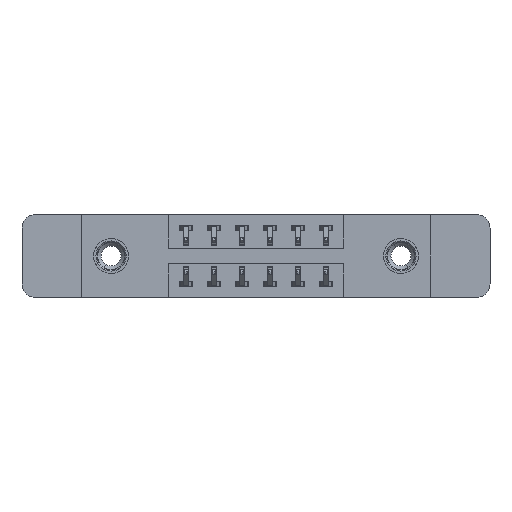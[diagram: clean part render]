
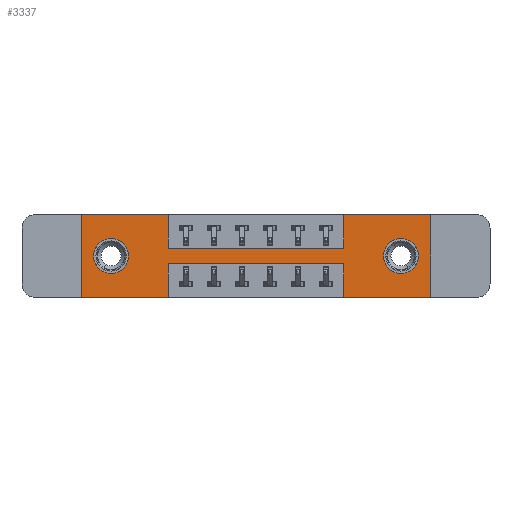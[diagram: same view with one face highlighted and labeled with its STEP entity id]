
A CAD part, front view. The second image highlights one B-rep face of the part: STEP entity #3337.
In plain terms, the highlighted planar face has unit normal (0, -1, 0).
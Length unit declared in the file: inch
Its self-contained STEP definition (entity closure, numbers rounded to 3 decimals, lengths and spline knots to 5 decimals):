
#36 = CARTESIAN_POINT ( 'NONE',  ( 1.1725, 0., -0.22 ) ) ;
#124 = AXIS2_PLACEMENT_3D ( 'NONE', #2717, #1734, #13635 ) ;
#217 = FACE_BOUND ( 'NONE', #1406, .T. ) ;
#240 = AXIS2_PLACEMENT_3D ( 'NONE', #813, #13958, #3029 ) ;
#244 = LINE ( 'NONE', #4098, #6102 ) ;
#320 = CARTESIAN_POINT ( 'NONE',  ( 1.1725, 0., -0.37 ) ) ;
#406 = LINE ( 'NONE', #913, #5225 ) ;
#577 = ORIENTED_EDGE ( 'NONE', *, *, #9553, .F. ) ;
#578 = CARTESIAN_POINT ( 'NONE',  ( 0., 0., -0.37 ) ) ;
#588 = LINE ( 'NONE', #1889, #13231 ) ;
#661 = LINE ( 'NONE', #10753, #5142 ) ;
#663 = ORIENTED_EDGE ( 'NONE', *, *, #7709, .F. ) ;
#774 = DIRECTION ( 'NONE',  ( 1., 0., 0. ) ) ;
#813 = CARTESIAN_POINT ( 'NONE',  ( 1.4275, 0., -0.185 ) ) ;
#877 = DIRECTION ( 'NONE',  ( 0., 0., 1. ) ) ;
#913 = CARTESIAN_POINT ( 'NONE',  ( 1.1725, 0., -0.37 ) ) ;
#930 = VECTOR ( 'NONE', #5246, 39.37008 ) ;
#980 = LINE ( 'NONE', #2436, #3235 ) ;
#1031 = DIRECTION ( 'NONE',  ( -1., 0., 0. ) ) ;
#1097 = LINE ( 'NONE', #12730, #930 ) ;
#1406 = EDGE_LOOP ( 'NONE', ( #3164, #3197 ) ) ;
#1559 = LINE ( 'NONE', #4220, #3796 ) ;
#1603 = PLANE ( 'NONE',  #124 ) ;
#1734 = DIRECTION ( 'NONE',  ( 0., -1., 0. ) ) ;
#1872 = EDGE_CURVE ( 'NONE', #7297, #12879, #4726, .T. ) ;
#1889 = CARTESIAN_POINT ( 'NONE',  ( 1.1725, 0., 0. ) ) ;
#2072 = VERTEX_POINT ( 'NONE', #320 ) ;
#2246 = VECTOR ( 'NONE', #11998, 39.37008 ) ;
#2436 = CARTESIAN_POINT ( 'NONE',  ( 0., 0., -0.37 ) ) ;
#2717 = CARTESIAN_POINT ( 'NONE',  ( 0., 0., -0.37 ) ) ;
#2757 = LINE ( 'NONE', #8033, #12459 ) ;
#2758 = CIRCLE ( 'NONE', #240, 0.078 ) ;
#2958 = VERTEX_POINT ( 'NONE', #13514 ) ;
#3029 = DIRECTION ( 'NONE',  ( 0., 0., -1. ) ) ;
#3122 = ORIENTED_EDGE ( 'NONE', *, *, #12775, .T. ) ;
#3164 = ORIENTED_EDGE ( 'NONE', *, *, #4506, .T. ) ;
#3196 = CARTESIAN_POINT ( 'NONE',  ( 0., 0., 0. ) ) ;
#3197 = ORIENTED_EDGE ( 'NONE', *, *, #11159, .T. ) ;
#3235 = VECTOR ( 'NONE', #7865, 39.37008 ) ;
#3301 = FACE_OUTER_BOUND ( 'NONE', #11328, .T. ) ;
#3337 = ADVANCED_FACE ( 'NONE', ( #217, #10773, #3301 ), #1603, .T. ) ;
#3426 = ORIENTED_EDGE ( 'NONE', *, *, #11419, .F. ) ;
#3471 = DIRECTION ( 'NONE',  ( 0., 1., 0. ) ) ;
#3548 = AXIS2_PLACEMENT_3D ( 'NONE', #3570, #13482, #5794 ) ;
#3570 = CARTESIAN_POINT ( 'NONE',  ( 1.4275, 0., -0.185 ) ) ;
#3595 = CARTESIAN_POINT ( 'NONE',  ( 1.1725, 0., -0.15 ) ) ;
#3692 = VECTOR ( 'NONE', #6111, 39.37008 ) ;
#3796 = VECTOR ( 'NONE', #12183, 39.37008 ) ;
#3921 = EDGE_CURVE ( 'NONE', #5388, #12815, #11264, .T. ) ;
#3966 = DIRECTION ( 'NONE',  ( 1., 0., 0. ) ) ;
#4052 = EDGE_CURVE ( 'NONE', #13413, #6311, #1559, .T. ) ;
#4098 = CARTESIAN_POINT ( 'NONE',  ( 0., 0., 0. ) ) ;
#4147 = CARTESIAN_POINT ( 'NONE',  ( 0.3875, 0., -0.37 ) ) ;
#4220 = CARTESIAN_POINT ( 'NONE',  ( 1.56, 0., 0. ) ) ;
#4366 = VERTEX_POINT ( 'NONE', #7771 ) ;
#4392 = CIRCLE ( 'NONE', #3548, 0.078 ) ;
#4485 = EDGE_CURVE ( 'NONE', #5446, #2958, #8741, .T. ) ;
#4506 = EDGE_CURVE ( 'NONE', #12605, #4366, #2758, .T. ) ;
#4726 = CIRCLE ( 'NONE', #9571, 0.078 ) ;
#4784 = CARTESIAN_POINT ( 'NONE',  ( 1.56, 0., -0.37 ) ) ;
#5142 = VECTOR ( 'NONE', #1031, 39.37008 ) ;
#5225 = VECTOR ( 'NONE', #10772, 39.37008 ) ;
#5246 = DIRECTION ( 'NONE',  ( 0., 0., -1. ) ) ;
#5388 = VERTEX_POINT ( 'NONE', #36 ) ;
#5446 = VERTEX_POINT ( 'NONE', #13851 ) ;
#5616 = VERTEX_POINT ( 'NONE', #3595 ) ;
#5794 = DIRECTION ( 'NONE',  ( 0., 0., -1. ) ) ;
#5885 = ORIENTED_EDGE ( 'NONE', *, *, #8871, .F. ) ;
#5951 = CARTESIAN_POINT ( 'NONE',  ( 0.3875, 0., 0. ) ) ;
#6102 = VECTOR ( 'NONE', #774, 39.37008 ) ;
#6111 = DIRECTION ( 'NONE',  ( 1., 0., 0. ) ) ;
#6289 = CARTESIAN_POINT ( 'NONE',  ( 0., 0., 0. ) ) ;
#6311 = VERTEX_POINT ( 'NONE', #4784 ) ;
#6320 = LINE ( 'NONE', #6289, #11874 ) ;
#6449 = CARTESIAN_POINT ( 'NONE',  ( 0.3875, 0., -0.22 ) ) ;
#6675 = ORIENTED_EDGE ( 'NONE', *, *, #4485, .F. ) ;
#6899 = ORIENTED_EDGE ( 'NONE', *, *, #8560, .F. ) ;
#7297 = VERTEX_POINT ( 'NONE', #13459 ) ;
#7414 = DIRECTION ( 'NONE',  ( 0., 0., -1. ) ) ;
#7482 = CARTESIAN_POINT ( 'NONE',  ( 0.1325, 0., -0.185 ) ) ;
#7622 = DIRECTION ( 'NONE',  ( 0., 0., 1. ) ) ;
#7688 = ORIENTED_EDGE ( 'NONE', *, *, #3921, .F. ) ;
#7709 = EDGE_CURVE ( 'NONE', #13594, #8801, #2757, .T. ) ;
#7771 = CARTESIAN_POINT ( 'NONE',  ( 1.4275, 0., -0.263 ) ) ;
#7865 = DIRECTION ( 'NONE',  ( -1., 0., 0. ) ) ;
#7995 = ORIENTED_EDGE ( 'NONE', *, *, #11277, .F. ) ;
#8033 = CARTESIAN_POINT ( 'NONE',  ( 0., 0., 0. ) ) ;
#8186 = CARTESIAN_POINT ( 'NONE',  ( 1.4275, 0., -0.107 ) ) ;
#8560 = EDGE_CURVE ( 'NONE', #11665, #13594, #661, .T. ) ;
#8741 = LINE ( 'NONE', #5951, #12954 ) ;
#8801 = VERTEX_POINT ( 'NONE', #3196 ) ;
#8808 = LINE ( 'NONE', #13654, #3692 ) ;
#8849 = AXIS2_PLACEMENT_3D ( 'NONE', #7482, #13144, #7622 ) ;
#8871 = EDGE_CURVE ( 'NONE', #6311, #2072, #980, .T. ) ;
#9462 = ORIENTED_EDGE ( 'NONE', *, *, #12743, .F. ) ;
#9553 = EDGE_CURVE ( 'NONE', #14010, #13413, #6320, .T. ) ;
#9571 = AXIS2_PLACEMENT_3D ( 'NONE', #9990, #3471, #10083 ) ;
#9990 = CARTESIAN_POINT ( 'NONE',  ( 0.1325, 0., -0.185 ) ) ;
#10083 = DIRECTION ( 'NONE',  ( 0., 0., 1. ) ) ;
#10331 = DIRECTION ( 'NONE',  ( 0., 0., 1. ) ) ;
#10675 = ORIENTED_EDGE ( 'NONE', *, *, #11649, .F. ) ;
#10753 = CARTESIAN_POINT ( 'NONE',  ( 0., 0., -0.37 ) ) ;
#10772 = DIRECTION ( 'NONE',  ( 0., 0., 1. ) ) ;
#10773 = FACE_BOUND ( 'NONE', #13080, .T. ) ;
#10951 = EDGE_CURVE ( 'NONE', #2958, #5616, #8808, .T. ) ;
#11159 = EDGE_CURVE ( 'NONE', #4366, #12605, #4392, .T. ) ;
#11168 = ORIENTED_EDGE ( 'NONE', *, *, #10951, .F. ) ;
#11264 = LINE ( 'NONE', #6449, #2246 ) ;
#11277 = EDGE_CURVE ( 'NONE', #12815, #11665, #1097, .T. ) ;
#11328 = EDGE_LOOP ( 'NONE', ( #7995, #7688, #10675, #5885, #12515, #577, #9462, #11168, #6675, #3426, #663, #6899 ) ) ;
#11330 = CIRCLE ( 'NONE', #8849, 0.078 ) ;
#11419 = EDGE_CURVE ( 'NONE', #8801, #5446, #244, .T. ) ;
#11649 = EDGE_CURVE ( 'NONE', #2072, #5388, #406, .T. ) ;
#11665 = VERTEX_POINT ( 'NONE', #4147 ) ;
#11874 = VECTOR ( 'NONE', #3966, 39.37008 ) ;
#11970 = CARTESIAN_POINT ( 'NONE',  ( 0.3875, 0., -0.22 ) ) ;
#11998 = DIRECTION ( 'NONE',  ( -1., 0., 0. ) ) ;
#12183 = DIRECTION ( 'NONE',  ( 0., 0., -1. ) ) ;
#12459 = VECTOR ( 'NONE', #10331, 39.37008 ) ;
#12515 = ORIENTED_EDGE ( 'NONE', *, *, #4052, .F. ) ;
#12533 = ORIENTED_EDGE ( 'NONE', *, *, #1872, .T. ) ;
#12605 = VERTEX_POINT ( 'NONE', #8186 ) ;
#12730 = CARTESIAN_POINT ( 'NONE',  ( 0.3875, 0., -0.37 ) ) ;
#12743 = EDGE_CURVE ( 'NONE', #5616, #14010, #588, .T. ) ;
#12775 = EDGE_CURVE ( 'NONE', #12879, #7297, #11330, .T. ) ;
#12815 = VERTEX_POINT ( 'NONE', #11970 ) ;
#12879 = VERTEX_POINT ( 'NONE', #14124 ) ;
#12954 = VECTOR ( 'NONE', #7414, 39.37008 ) ;
#13080 = EDGE_LOOP ( 'NONE', ( #3122, #12533 ) ) ;
#13109 = CARTESIAN_POINT ( 'NONE',  ( 1.1725, 0., 0. ) ) ;
#13144 = DIRECTION ( 'NONE',  ( 0., 1., 0. ) ) ;
#13231 = VECTOR ( 'NONE', #877, 39.37008 ) ;
#13413 = VERTEX_POINT ( 'NONE', #13916 ) ;
#13459 = CARTESIAN_POINT ( 'NONE',  ( 0.1325, 0., -0.263 ) ) ;
#13482 = DIRECTION ( 'NONE',  ( 0., 1., 0. ) ) ;
#13514 = CARTESIAN_POINT ( 'NONE',  ( 0.3875, 0., -0.15 ) ) ;
#13594 = VERTEX_POINT ( 'NONE', #578 ) ;
#13635 = DIRECTION ( 'NONE',  ( 0., 0., -1. ) ) ;
#13654 = CARTESIAN_POINT ( 'NONE',  ( 0.3875, 0., -0.15 ) ) ;
#13851 = CARTESIAN_POINT ( 'NONE',  ( 0.3875, 0., 0. ) ) ;
#13916 = CARTESIAN_POINT ( 'NONE',  ( 1.56, 0., 0. ) ) ;
#13958 = DIRECTION ( 'NONE',  ( 0., 1., 0. ) ) ;
#14010 = VERTEX_POINT ( 'NONE', #13109 ) ;
#14124 = CARTESIAN_POINT ( 'NONE',  ( 0.1325, 0., -0.107 ) ) ;
